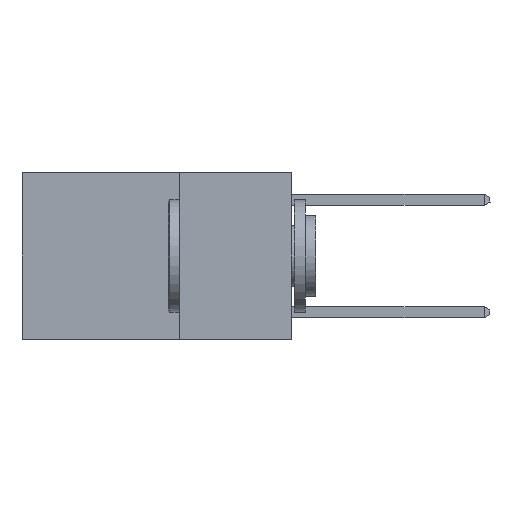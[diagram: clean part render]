
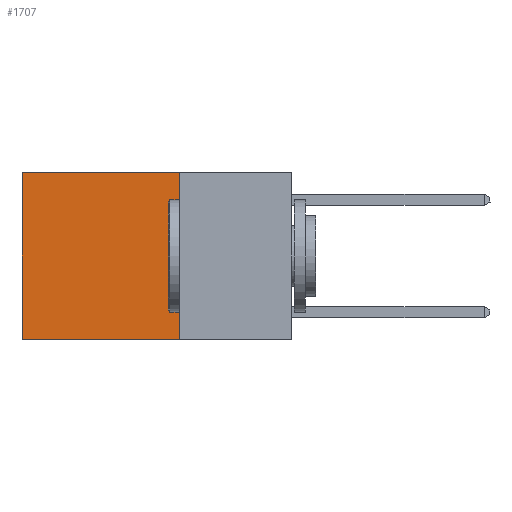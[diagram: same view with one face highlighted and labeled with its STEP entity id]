
A CAD part, left-side view. The second image highlights one B-rep face of the part: STEP entity #1707.
In plain terms, the highlighted planar face has unit normal (-1, 0, 0).
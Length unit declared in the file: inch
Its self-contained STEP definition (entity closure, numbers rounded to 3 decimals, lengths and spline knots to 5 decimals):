
#9 = VERTEX_POINT ( 'NONE', #7661 ) ;
#99 = EDGE_CURVE ( 'NONE', #8656, #11278, #9826, .T. ) ;
#496 = DIRECTION ( 'NONE',  ( 0., 0., -1. ) ) ;
#1100 = ORIENTED_EDGE ( 'NONE', *, *, #4456, .F. ) ;
#1690 = AXIS2_PLACEMENT_3D ( 'NONE', #16070, #9090, #496 ) ;
#1707 = ADVANCED_FACE ( 'NONE', ( #17363 ), #11893, .F. ) ;
#1776 = LINE ( 'NONE', #18181, #16413 ) ;
#2022 = ORIENTED_EDGE ( 'NONE', *, *, #10527, .T. ) ;
#4456 = EDGE_CURVE ( 'NONE', #9, #11278, #1776, .T. ) ;
#4633 = CARTESIAN_POINT ( 'NONE',  ( 0.2625, 0.6, 0. ) ) ;
#4788 = VECTOR ( 'NONE', #9544, 39.37008 ) ;
#6002 = CARTESIAN_POINT ( 'NONE',  ( 0.2625, 0.25, 0. ) ) ;
#6077 = VECTOR ( 'NONE', #11654, 39.37008 ) ;
#6606 = ORIENTED_EDGE ( 'NONE', *, *, #99, .T. ) ;
#7463 = EDGE_LOOP ( 'NONE', ( #6606, #1100, #14158, #2022 ) ) ;
#7661 = CARTESIAN_POINT ( 'NONE',  ( 0.2625, 0.25, -0.37 ) ) ;
#7887 = LINE ( 'NONE', #12433, #14907 ) ;
#8656 = VERTEX_POINT ( 'NONE', #4633 ) ;
#9090 = DIRECTION ( 'NONE',  ( 1., 0., 0. ) ) ;
#9544 = DIRECTION ( 'NONE',  ( 0., 1., 0. ) ) ;
#9826 = LINE ( 'NONE', #17046, #6077 ) ;
#10527 = EDGE_CURVE ( 'NONE', #11290, #8656, #12334, .T. ) ;
#11278 = VERTEX_POINT ( 'NONE', #13063 ) ;
#11290 = VERTEX_POINT ( 'NONE', #6002 ) ;
#11321 = DIRECTION ( 'NONE',  ( 0., 1., 0. ) ) ;
#11654 = DIRECTION ( 'NONE',  ( 0., 0., -1. ) ) ;
#11665 = EDGE_CURVE ( 'NONE', #11290, #9, #7887, .T. ) ;
#11893 = PLANE ( 'NONE',  #1690 ) ;
#12334 = LINE ( 'NONE', #15183, #4788 ) ;
#12433 = CARTESIAN_POINT ( 'NONE',  ( 0.2625, 0.25, 0. ) ) ;
#13063 = CARTESIAN_POINT ( 'NONE',  ( 0.2625, 0.6, -0.37 ) ) ;
#14158 = ORIENTED_EDGE ( 'NONE', *, *, #11665, .F. ) ;
#14907 = VECTOR ( 'NONE', #17961, 39.37008 ) ;
#15183 = CARTESIAN_POINT ( 'NONE',  ( 0.2625, 0.25, 0. ) ) ;
#16070 = CARTESIAN_POINT ( 'NONE',  ( 0.2625, 0.25, 0. ) ) ;
#16413 = VECTOR ( 'NONE', #11321, 39.37008 ) ;
#17046 = CARTESIAN_POINT ( 'NONE',  ( 0.2625, 0.6, 0. ) ) ;
#17363 = FACE_OUTER_BOUND ( 'NONE', #7463, .T. ) ;
#17961 = DIRECTION ( 'NONE',  ( 0., 0., -1. ) ) ;
#18181 = CARTESIAN_POINT ( 'NONE',  ( 0.2625, 0.25, -0.37 ) ) ;
